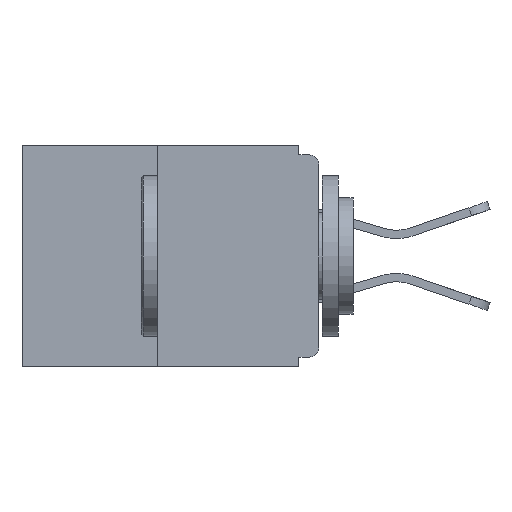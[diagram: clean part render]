
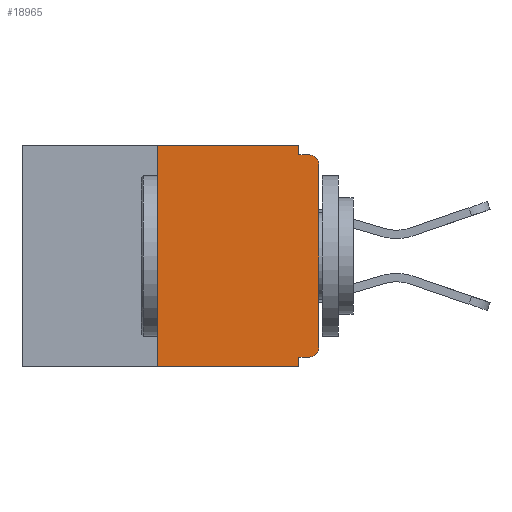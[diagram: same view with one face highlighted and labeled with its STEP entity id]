
A CAD part, left-side view. The second image highlights one B-rep face of the part: STEP entity #18965.
In plain terms, the highlighted planar face has unit normal (-1, 0, 0).
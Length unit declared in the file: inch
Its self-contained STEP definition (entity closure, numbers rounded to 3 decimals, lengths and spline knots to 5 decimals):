
#12 = CARTESIAN_POINT ( 'NONE',  ( 0., 0.015, -0.328 ) ) ;
#69 = DIRECTION ( 'NONE',  ( 0., 0., 1. ) ) ;
#85 = CARTESIAN_POINT ( 'NONE',  ( 0., 0.46, 0. ) ) ;
#594 = VERTEX_POINT ( 'NONE', #6495 ) ;
#1378 = VECTOR ( 'NONE', #13889, 39.37008 ) ;
#2071 = ORIENTED_EDGE ( 'NONE', *, *, #5933, .F. ) ;
#2267 = VERTEX_POINT ( 'NONE', #11676 ) ;
#2560 = EDGE_CURVE ( 'NONE', #16620, #6023, #11050, .T. ) ;
#2614 = LINE ( 'NONE', #9958, #13145 ) ;
#2675 = VECTOR ( 'NONE', #4266, 39.37008 ) ;
#2813 = EDGE_CURVE ( 'NONE', #6023, #594, #4628, .T. ) ;
#3210 = EDGE_CURVE ( 'NONE', #4343, #8362, #9103, .T. ) ;
#3212 = LINE ( 'NONE', #13945, #12088 ) ;
#3587 = EDGE_CURVE ( 'NONE', #17464, #4343, #3212, .T. ) ;
#3854 = LINE ( 'NONE', #6530, #17475 ) ;
#4138 = CARTESIAN_POINT ( 'NONE',  ( 0., 0.015, -0.03 ) ) ;
#4158 = EDGE_CURVE ( 'NONE', #2267, #594, #2614, .T. ) ;
#4266 = DIRECTION ( 'NONE',  ( 0., 0., -1. ) ) ;
#4343 = VERTEX_POINT ( 'NONE', #13421 ) ;
#4628 = LINE ( 'NONE', #18571, #2675 ) ;
#5183 = CARTESIAN_POINT ( 'NONE',  ( 0., 0., -0.03 ) ) ;
#5318 = ORIENTED_EDGE ( 'NONE', *, *, #10974, .T. ) ;
#5331 = LINE ( 'NONE', #19502, #1378 ) ;
#5933 = EDGE_CURVE ( 'NONE', #8362, #18317, #5331, .T. ) ;
#6023 = VERTEX_POINT ( 'NONE', #16172 ) ;
#6495 = CARTESIAN_POINT ( 'NONE',  ( 0., 0.031, -0.343 ) ) ;
#6530 = CARTESIAN_POINT ( 'NONE',  ( 0., 0., 0. ) ) ;
#6643 = CARTESIAN_POINT ( 'NONE',  ( 0., 0., -0.328 ) ) ;
#6778 = CARTESIAN_POINT ( 'NONE',  ( 0., 0., -0.313 ) ) ;
#6798 = CARTESIAN_POINT ( 'NONE',  ( 0., 0.015, -0.015 ) ) ;
#7741 = VECTOR ( 'NONE', #16015, 39.37008 ) ;
#8102 = DIRECTION ( 'NONE',  ( 0., 0., 1. ) ) ;
#8362 = VERTEX_POINT ( 'NONE', #14863 ) ;
#8462 = CARTESIAN_POINT ( 'NONE',  ( 0., 0.25, 0. ) ) ;
#8660 = DIRECTION ( 'NONE',  ( 0., -1., 0. ) ) ;
#8750 = CARTESIAN_POINT ( 'NONE',  ( 0., 0.015, -0.313 ) ) ;
#8997 = EDGE_CURVE ( 'NONE', #10694, #16907, #3854, .T. ) ;
#9103 = LINE ( 'NONE', #19167, #10754 ) ;
#9515 = EDGE_CURVE ( 'NONE', #2267, #17464, #13768, .T. ) ;
#9958 = CARTESIAN_POINT ( 'NONE',  ( 0., 0.46, -0.343 ) ) ;
#10352 = EDGE_CURVE ( 'NONE', #16907, #18317, #11821, .T. ) ;
#10694 = VERTEX_POINT ( 'NONE', #6778 ) ;
#10754 = VECTOR ( 'NONE', #18932, 39.37008 ) ;
#10974 = EDGE_CURVE ( 'NONE', #16620, #10694, #21661, .T. ) ;
#11050 = LINE ( 'NONE', #6643, #7741 ) ;
#11467 = ORIENTED_EDGE ( 'NONE', *, *, #3587, .F. ) ;
#11594 = DIRECTION ( 'NONE',  ( -1., 0., 0. ) ) ;
#11676 = CARTESIAN_POINT ( 'NONE',  ( 0., 0.25, -0.343 ) ) ;
#11821 = CIRCLE ( 'NONE', #20298, 0.015 ) ;
#12088 = VECTOR ( 'NONE', #8660, 39.37008 ) ;
#12400 = DIRECTION ( 'NONE',  ( 1., 0., 0. ) ) ;
#13145 = VECTOR ( 'NONE', #20937, 39.37008 ) ;
#13421 = CARTESIAN_POINT ( 'NONE',  ( 0., 0.031, 0. ) ) ;
#13569 = DIRECTION ( 'NONE',  ( -1., 0., 0. ) ) ;
#13768 = LINE ( 'NONE', #8462, #19140 ) ;
#13889 = DIRECTION ( 'NONE',  ( 0., -1., 0. ) ) ;
#13940 = AXIS2_PLACEMENT_3D ( 'NONE', #85, #12400, #15972 ) ;
#13945 = CARTESIAN_POINT ( 'NONE',  ( 0., 0.46, 0. ) ) ;
#13979 = AXIS2_PLACEMENT_3D ( 'NONE', #8750, #11594, #16165 ) ;
#14141 = ORIENTED_EDGE ( 'NONE', *, *, #4158, .T. ) ;
#14527 = ORIENTED_EDGE ( 'NONE', *, *, #3210, .F. ) ;
#14564 = ORIENTED_EDGE ( 'NONE', *, *, #10352, .T. ) ;
#14863 = CARTESIAN_POINT ( 'NONE',  ( 0., 0.031, -0.015 ) ) ;
#15542 = EDGE_LOOP ( 'NONE', ( #11467, #21960, #14141, #16639, #19842, #5318, #15724, #14564, #2071, #14527 ) ) ;
#15724 = ORIENTED_EDGE ( 'NONE', *, *, #8997, .T. ) ;
#15972 = DIRECTION ( 'NONE',  ( 0., 0., -1. ) ) ;
#16015 = DIRECTION ( 'NONE',  ( 0., 1., 0. ) ) ;
#16165 = DIRECTION ( 'NONE',  ( 0., 0., -1. ) ) ;
#16172 = CARTESIAN_POINT ( 'NONE',  ( 0., 0.031, -0.328 ) ) ;
#16620 = VERTEX_POINT ( 'NONE', #12 ) ;
#16639 = ORIENTED_EDGE ( 'NONE', *, *, #2813, .F. ) ;
#16907 = VERTEX_POINT ( 'NONE', #5183 ) ;
#17464 = VERTEX_POINT ( 'NONE', #21781 ) ;
#17475 = VECTOR ( 'NONE', #8102, 39.37008 ) ;
#18317 = VERTEX_POINT ( 'NONE', #6798 ) ;
#18571 = CARTESIAN_POINT ( 'NONE',  ( 0., 0.031, -0.343 ) ) ;
#18932 = DIRECTION ( 'NONE',  ( 0., 0., -1. ) ) ;
#18965 = ADVANCED_FACE ( 'NONE', ( #22718 ), #21348, .F. ) ;
#19140 = VECTOR ( 'NONE', #69, 39.37008 ) ;
#19167 = CARTESIAN_POINT ( 'NONE',  ( 0., 0.031, 0. ) ) ;
#19502 = CARTESIAN_POINT ( 'NONE',  ( 0., 0., -0.015 ) ) ;
#19842 = ORIENTED_EDGE ( 'NONE', *, *, #2560, .F. ) ;
#20208 = DIRECTION ( 'NONE',  ( 0., 0., -1. ) ) ;
#20298 = AXIS2_PLACEMENT_3D ( 'NONE', #4138, #13569, #20208 ) ;
#20937 = DIRECTION ( 'NONE',  ( 0., -1., 0. ) ) ;
#21348 = PLANE ( 'NONE',  #13940 ) ;
#21661 = CIRCLE ( 'NONE', #13979, 0.015 ) ;
#21781 = CARTESIAN_POINT ( 'NONE',  ( 0., 0.25, 0. ) ) ;
#21960 = ORIENTED_EDGE ( 'NONE', *, *, #9515, .F. ) ;
#22718 = FACE_OUTER_BOUND ( 'NONE', #15542, .T. ) ;
